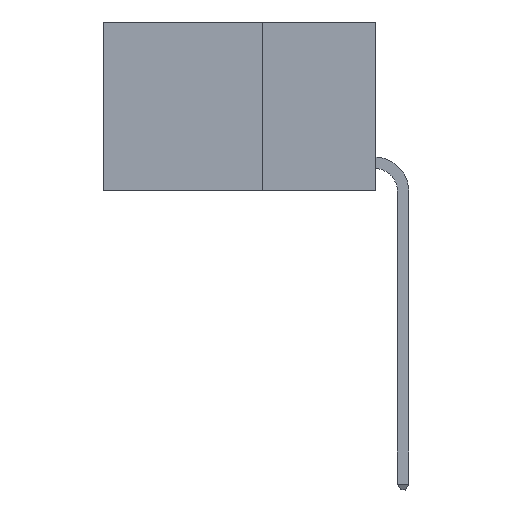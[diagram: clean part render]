
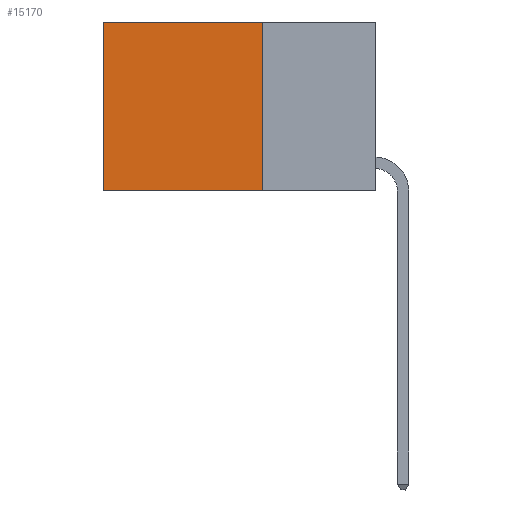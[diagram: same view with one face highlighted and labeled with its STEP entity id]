
A CAD part, left-side view. The second image highlights one B-rep face of the part: STEP entity #15170.
In plain terms, the highlighted planar face has unit normal (-1, 0, 0).
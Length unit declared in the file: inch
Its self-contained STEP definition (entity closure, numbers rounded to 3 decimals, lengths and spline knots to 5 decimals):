
#405 = ORIENTED_EDGE ( 'NONE', *, *, #2228, .F. ) ;
#1797 = VERTEX_POINT ( 'NONE', #14490 ) ;
#2099 = LINE ( 'NONE', #13503, #15231 ) ;
#2228 = EDGE_CURVE ( 'NONE', #8172, #10137, #13475, .T. ) ;
#2901 = CARTESIAN_POINT ( 'NONE',  ( 0.2625, 0.6, 0. ) ) ;
#3954 = EDGE_CURVE ( 'NONE', #13012, #8172, #5951, .T. ) ;
#4184 = DIRECTION ( 'NONE',  ( 0., 0., -1. ) ) ;
#4757 = CARTESIAN_POINT ( 'NONE',  ( 0.2625, 0.25, 0. ) ) ;
#5479 = ORIENTED_EDGE ( 'NONE', *, *, #3954, .F. ) ;
#5684 = EDGE_CURVE ( 'NONE', #1797, #10137, #11737, .T. ) ;
#5944 = CARTESIAN_POINT ( 'NONE',  ( 0.2625, 0.25, -0.37 ) ) ;
#5951 = LINE ( 'NONE', #14910, #12063 ) ;
#5978 = ORIENTED_EDGE ( 'NONE', *, *, #13393, .T. ) ;
#6180 = DIRECTION ( 'NONE',  ( 0., 1., 0. ) ) ;
#7250 = PLANE ( 'NONE',  #15781 ) ;
#7565 = EDGE_LOOP ( 'NONE', ( #10192, #405, #5479, #5978 ) ) ;
#8172 = VERTEX_POINT ( 'NONE', #5944 ) ;
#8472 = VECTOR ( 'NONE', #4184, 39.37008 ) ;
#8476 = DIRECTION ( 'NONE',  ( 0., 0., -1. ) ) ;
#10137 = VERTEX_POINT ( 'NONE', #12712 ) ;
#10192 = ORIENTED_EDGE ( 'NONE', *, *, #5684, .T. ) ;
#10250 = VECTOR ( 'NONE', #14778, 39.37008 ) ;
#11737 = LINE ( 'NONE', #2901, #8472 ) ;
#12063 = VECTOR ( 'NONE', #13258, 39.37008 ) ;
#12712 = CARTESIAN_POINT ( 'NONE',  ( 0.2625, 0.6, -0.37 ) ) ;
#13012 = VERTEX_POINT ( 'NONE', #14055 ) ;
#13258 = DIRECTION ( 'NONE',  ( 0., 0., -1. ) ) ;
#13393 = EDGE_CURVE ( 'NONE', #13012, #1797, #2099, .T. ) ;
#13475 = LINE ( 'NONE', #15329, #10250 ) ;
#13503 = CARTESIAN_POINT ( 'NONE',  ( 0.2625, 0.25, 0. ) ) ;
#14055 = CARTESIAN_POINT ( 'NONE',  ( 0.2625, 0.25, 0. ) ) ;
#14490 = CARTESIAN_POINT ( 'NONE',  ( 0.2625, 0.6, 0. ) ) ;
#14778 = DIRECTION ( 'NONE',  ( 0., 1., 0. ) ) ;
#14910 = CARTESIAN_POINT ( 'NONE',  ( 0.2625, 0.25, 0. ) ) ;
#15170 = ADVANCED_FACE ( 'NONE', ( #15176 ), #7250, .F. ) ;
#15176 = FACE_OUTER_BOUND ( 'NONE', #7565, .T. ) ;
#15231 = VECTOR ( 'NONE', #6180, 39.37008 ) ;
#15329 = CARTESIAN_POINT ( 'NONE',  ( 0.2625, 0.25, -0.37 ) ) ;
#15767 = DIRECTION ( 'NONE',  ( 1., 0., 0. ) ) ;
#15781 = AXIS2_PLACEMENT_3D ( 'NONE', #4757, #15767, #8476 ) ;
